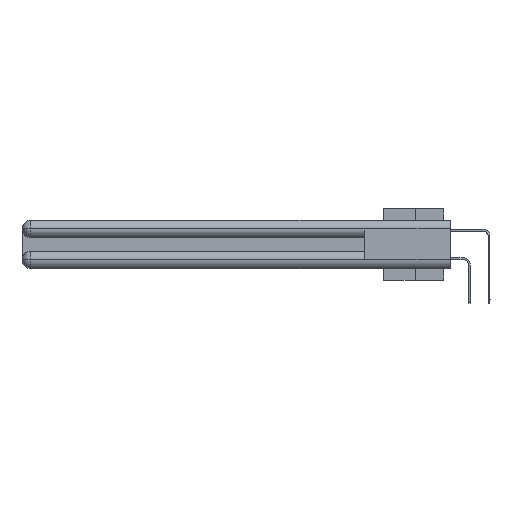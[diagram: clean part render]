
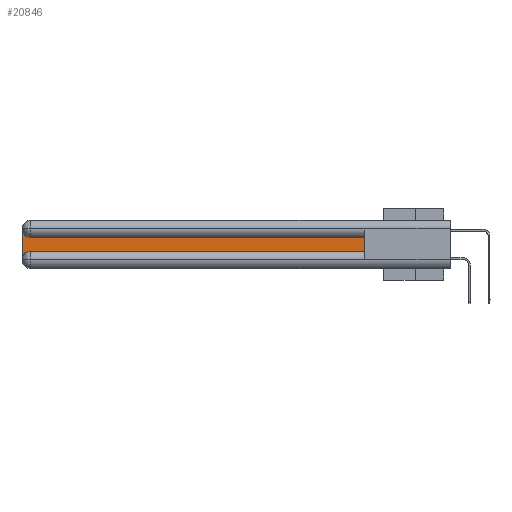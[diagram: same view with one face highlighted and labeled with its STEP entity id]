
A CAD part, left-side view. The second image highlights one B-rep face of the part: STEP entity #20846.
In plain terms, the highlighted planar face has unit normal (-1, 0, 0).
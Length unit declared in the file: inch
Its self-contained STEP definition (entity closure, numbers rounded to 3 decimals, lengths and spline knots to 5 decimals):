
#653 = VECTOR ( 'NONE', #36220, 39.37008 ) ;
#705 = DIRECTION ( 'NONE',  ( 0., 0., -1. ) ) ;
#967 = VECTOR ( 'NONE', #31371, 39.37008 ) ;
#1055 = ORIENTED_EDGE ( 'NONE', *, *, #5237, .T. ) ;
#1387 = CARTESIAN_POINT ( 'NONE',  ( 0.075, 3., -0.0625 ) ) ;
#2090 = VERTEX_POINT ( 'NONE', #1387 ) ;
#2250 = DIRECTION ( 'NONE',  ( 0., 0., -1. ) ) ;
#2498 = DIRECTION ( 'NONE',  ( 1., 0., 0. ) ) ;
#2756 = EDGE_LOOP ( 'NONE', ( #25976, #14764, #30355, #20612, #1055, #21318 ) ) ;
#5237 = EDGE_CURVE ( 'NONE', #13996, #19374, #26006, .T. ) ;
#5787 = DIRECTION ( 'NONE',  ( 1., 0., 0. ) ) ;
#5853 = LINE ( 'NONE', #30039, #11890 ) ;
#8422 = CIRCLE ( 'NONE', #33850, 0.06 ) ;
#8652 = DIRECTION ( 'NONE',  ( 0., 0., 1. ) ) ;
#8805 = AXIS2_PLACEMENT_3D ( 'NONE', #23713, #2498, #14591 ) ;
#8842 = CARTESIAN_POINT ( 'NONE',  ( 0.075, 2.94, -0.2175 ) ) ;
#10391 = CARTESIAN_POINT ( 'NONE',  ( 0.075, 0.6, -0.1225 ) ) ;
#11705 = EDGE_CURVE ( 'NONE', #19374, #13021, #5853, .T. ) ;
#11890 = VECTOR ( 'NONE', #8652, 39.37008 ) ;
#12192 = PLANE ( 'NONE',  #8805 ) ;
#13021 = VERTEX_POINT ( 'NONE', #27160 ) ;
#13996 = VERTEX_POINT ( 'NONE', #8842 ) ;
#14591 = DIRECTION ( 'NONE',  ( 0., 0., -1. ) ) ;
#14764 = ORIENTED_EDGE ( 'NONE', *, *, #27751, .T. ) ;
#17393 = AXIS2_PLACEMENT_3D ( 'NONE', #32815, #36352, #17756 ) ;
#17756 = DIRECTION ( 'NONE',  ( 0., 0., -1. ) ) ;
#18762 = CARTESIAN_POINT ( 'NONE',  ( 0.075, 3., -0.2175 ) ) ;
#19374 = VERTEX_POINT ( 'NONE', #32671 ) ;
#20612 = ORIENTED_EDGE ( 'NONE', *, *, #28214, .T. ) ;
#20828 = VERTEX_POINT ( 'NONE', #24284 ) ;
#20846 = ADVANCED_FACE ( 'NONE', ( #33219 ), #12192, .F. ) ;
#21318 = ORIENTED_EDGE ( 'NONE', *, *, #11705, .T. ) ;
#22196 = EDGE_CURVE ( 'NONE', #13021, #20828, #37532, .T. ) ;
#22849 = CARTESIAN_POINT ( 'NONE',  ( 0.075, 0.6, -0.2175 ) ) ;
#23713 = CARTESIAN_POINT ( 'NONE',  ( 0.075, 3., -0.1225 ) ) ;
#23987 = EDGE_CURVE ( 'NONE', #2090, #33387, #30627, .T. ) ;
#24284 = CARTESIAN_POINT ( 'NONE',  ( 0.075, 2.94, -0.1225 ) ) ;
#25976 = ORIENTED_EDGE ( 'NONE', *, *, #22196, .T. ) ;
#26006 = LINE ( 'NONE', #22849, #967 ) ;
#27160 = CARTESIAN_POINT ( 'NONE',  ( 0.075, 0.6, -0.1225 ) ) ;
#27241 = VECTOR ( 'NONE', #705, 39.37008 ) ;
#27751 = EDGE_CURVE ( 'NONE', #20828, #2090, #38239, .T. ) ;
#28214 = EDGE_CURVE ( 'NONE', #33387, #13996, #8422, .T. ) ;
#29390 = CARTESIAN_POINT ( 'NONE',  ( 0.075, 2.94, -0.2775 ) ) ;
#30039 = CARTESIAN_POINT ( 'NONE',  ( 0.075, 0.6, -0.2175 ) ) ;
#30355 = ORIENTED_EDGE ( 'NONE', *, *, #23987, .T. ) ;
#30627 = LINE ( 'NONE', #18762, #27241 ) ;
#31371 = DIRECTION ( 'NONE',  ( 0., -1., 0. ) ) ;
#32671 = CARTESIAN_POINT ( 'NONE',  ( 0.075, 0.6, -0.2175 ) ) ;
#32815 = CARTESIAN_POINT ( 'NONE',  ( 0.075, 2.94, -0.0625 ) ) ;
#33219 = FACE_OUTER_BOUND ( 'NONE', #2756, .T. ) ;
#33387 = VERTEX_POINT ( 'NONE', #34704 ) ;
#33850 = AXIS2_PLACEMENT_3D ( 'NONE', #29390, #5787, #2250 ) ;
#34704 = CARTESIAN_POINT ( 'NONE',  ( 0.075, 3., -0.2775 ) ) ;
#36220 = DIRECTION ( 'NONE',  ( 0., 1., 0. ) ) ;
#36352 = DIRECTION ( 'NONE',  ( 1., 0., 0. ) ) ;
#37532 = LINE ( 'NONE', #10391, #653 ) ;
#38239 = CIRCLE ( 'NONE', #17393, 0.06 ) ;
